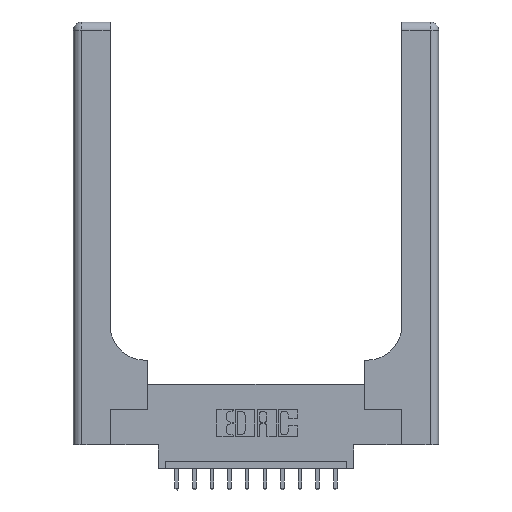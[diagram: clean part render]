
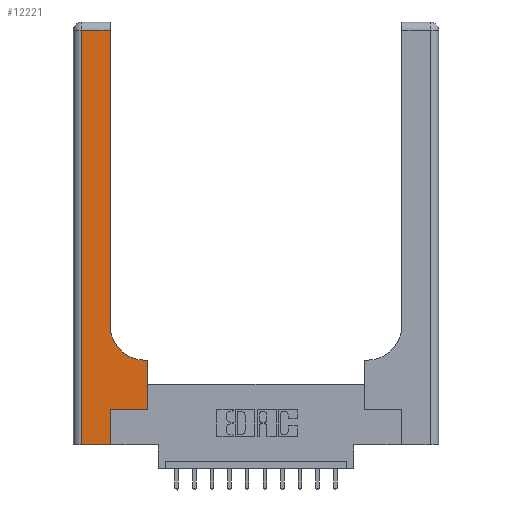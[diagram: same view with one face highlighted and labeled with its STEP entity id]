
A CAD part, top view. The second image highlights one B-rep face of the part: STEP entity #12221.
In plain terms, the highlighted planar face has unit normal (0, 0, 1).
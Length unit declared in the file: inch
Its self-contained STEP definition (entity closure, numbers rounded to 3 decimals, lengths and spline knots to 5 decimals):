
#10 = CARTESIAN_POINT ( 'NONE',  ( 0.528, 0.25, 0.37 ) ) ;
#270 = LINE ( 'NONE', #9635, #12931 ) ;
#585 = EDGE_CURVE ( 'NONE', #4422, #7403, #695, .T. ) ;
#695 = LINE ( 'NONE', #13138, #5099 ) ;
#870 = PLANE ( 'NONE',  #9956 ) ;
#887 = ORIENTED_EDGE ( 'NONE', *, *, #14950, .T. ) ;
#1253 = EDGE_LOOP ( 'NONE', ( #12838, #12222, #887, #7205, #13169, #4677, #11726, #8323, #15021 ) ) ;
#1298 = CIRCLE ( 'NONE', #12936, 0.25 ) ;
#1311 = EDGE_CURVE ( 'NONE', #8933, #1367, #7366, .T. ) ;
#1367 = VERTEX_POINT ( 'NONE', #2426 ) ;
#1423 = CARTESIAN_POINT ( 'NONE',  ( 0.528, 0.25, 0.37 ) ) ;
#1638 = DIRECTION ( 'NONE',  ( -1., 0., 0. ) ) ;
#2054 = FACE_OUTER_BOUND ( 'NONE', #1253, .T. ) ;
#2079 = CARTESIAN_POINT ( 'NONE',  ( 0.26, 3., 0.37 ) ) ;
#2120 = CARTESIAN_POINT ( 'NONE',  ( 0.51, 0.85, 0.37 ) ) ;
#2426 = CARTESIAN_POINT ( 'NONE',  ( 0.528, 0.6, 0.37 ) ) ;
#3192 = VERTEX_POINT ( 'NONE', #5986 ) ;
#3507 = VECTOR ( 'NONE', #1638, 39.37008 ) ;
#4422 = VERTEX_POINT ( 'NONE', #15256 ) ;
#4677 = ORIENTED_EDGE ( 'NONE', *, *, #9772, .T. ) ;
#5099 = VECTOR ( 'NONE', #12015, 39.37008 ) ;
#5582 = VERTEX_POINT ( 'NONE', #9370 ) ;
#5591 = CARTESIAN_POINT ( 'NONE',  ( 0.265, 0., 0.37 ) ) ;
#5759 = LINE ( 'NONE', #10356, #3507 ) ;
#5766 = VECTOR ( 'NONE', #14462, 39.37008 ) ;
#5986 = CARTESIAN_POINT ( 'NONE',  ( 0.06, 0., 0.37 ) ) ;
#5996 = CARTESIAN_POINT ( 'NONE',  ( 0.06, 3., 0.37 ) ) ;
#6014 = EDGE_CURVE ( 'NONE', #1367, #14629, #5759, .T. ) ;
#6108 = CARTESIAN_POINT ( 'NONE',  ( 0.26, 0.85, 0.37 ) ) ;
#6456 = LINE ( 'NONE', #2079, #10697 ) ;
#6844 = VECTOR ( 'NONE', #12197, 39.37008 ) ;
#7205 = ORIENTED_EDGE ( 'NONE', *, *, #11830, .T. ) ;
#7366 = LINE ( 'NONE', #10, #8142 ) ;
#7403 = VERTEX_POINT ( 'NONE', #12472 ) ;
#8084 = DIRECTION ( 'NONE',  ( 1., 0., 0. ) ) ;
#8142 = VECTOR ( 'NONE', #13253, 39.37008 ) ;
#8323 = ORIENTED_EDGE ( 'NONE', *, *, #6014, .T. ) ;
#8553 = VECTOR ( 'NONE', #8084, 39.37008 ) ;
#8602 = CARTESIAN_POINT ( 'NONE',  ( 0., 0., 0.37 ) ) ;
#8771 = LINE ( 'NONE', #8602, #6844 ) ;
#8779 = EDGE_CURVE ( 'NONE', #9436, #4422, #6456, .T. ) ;
#8933 = VERTEX_POINT ( 'NONE', #1423 ) ;
#9281 = CARTESIAN_POINT ( 'NONE',  ( 0., 3., 0.37 ) ) ;
#9370 = CARTESIAN_POINT ( 'NONE',  ( 0.265, 0.25, 0.37 ) ) ;
#9436 = VERTEX_POINT ( 'NONE', #6108 ) ;
#9448 = DIRECTION ( 'NONE',  ( -1., 0., 0. ) ) ;
#9532 = DIRECTION ( 'NONE',  ( 0., 1., 0. ) ) ;
#9635 = CARTESIAN_POINT ( 'NONE',  ( 0.265, 0., 0.37 ) ) ;
#9772 = EDGE_CURVE ( 'NONE', #5582, #8933, #11817, .T. ) ;
#9956 = AXIS2_PLACEMENT_3D ( 'NONE', #9281, #13040, #9448 ) ;
#10347 = CARTESIAN_POINT ( 'NONE',  ( 0.51, 0.6, 0.37 ) ) ;
#10356 = CARTESIAN_POINT ( 'NONE',  ( 0.26, 0.6, 0.37 ) ) ;
#10697 = VECTOR ( 'NONE', #12253, 39.37008 ) ;
#10702 = DIRECTION ( 'NONE',  ( 1., 0., 0. ) ) ;
#10805 = DIRECTION ( 'NONE',  ( 0., 0., -1. ) ) ;
#11684 = EDGE_CURVE ( 'NONE', #14629, #9436, #1298, .T. ) ;
#11726 = ORIENTED_EDGE ( 'NONE', *, *, #1311, .T. ) ;
#11817 = LINE ( 'NONE', #15560, #8553 ) ;
#11830 = EDGE_CURVE ( 'NONE', #3192, #13581, #8771, .T. ) ;
#12015 = DIRECTION ( 'NONE',  ( -1., 0., 0. ) ) ;
#12197 = DIRECTION ( 'NONE',  ( 1., 0., 0. ) ) ;
#12221 = ADVANCED_FACE ( 'NONE', ( #2054 ), #870, .F. ) ;
#12222 = ORIENTED_EDGE ( 'NONE', *, *, #585, .T. ) ;
#12253 = DIRECTION ( 'NONE',  ( 0., 1., 0. ) ) ;
#12472 = CARTESIAN_POINT ( 'NONE',  ( 0.06, 2.94, 0.37 ) ) ;
#12695 = LINE ( 'NONE', #5996, #5766 ) ;
#12838 = ORIENTED_EDGE ( 'NONE', *, *, #8779, .T. ) ;
#12931 = VECTOR ( 'NONE', #9532, 39.37008 ) ;
#12936 = AXIS2_PLACEMENT_3D ( 'NONE', #2120, #10805, #10702 ) ;
#13040 = DIRECTION ( 'NONE',  ( 0., 0., -1. ) ) ;
#13138 = CARTESIAN_POINT ( 'NONE',  ( 0., 2.94, 0.37 ) ) ;
#13169 = ORIENTED_EDGE ( 'NONE', *, *, #13690, .T. ) ;
#13253 = DIRECTION ( 'NONE',  ( 0., 1., 0. ) ) ;
#13581 = VERTEX_POINT ( 'NONE', #5591 ) ;
#13690 = EDGE_CURVE ( 'NONE', #13581, #5582, #270, .T. ) ;
#14462 = DIRECTION ( 'NONE',  ( 0., -1., 0. ) ) ;
#14629 = VERTEX_POINT ( 'NONE', #10347 ) ;
#14950 = EDGE_CURVE ( 'NONE', #7403, #3192, #12695, .T. ) ;
#15021 = ORIENTED_EDGE ( 'NONE', *, *, #11684, .T. ) ;
#15256 = CARTESIAN_POINT ( 'NONE',  ( 0.26, 2.94, 0.37 ) ) ;
#15560 = CARTESIAN_POINT ( 'NONE',  ( 0.265, 0.25, 0.37 ) ) ;
